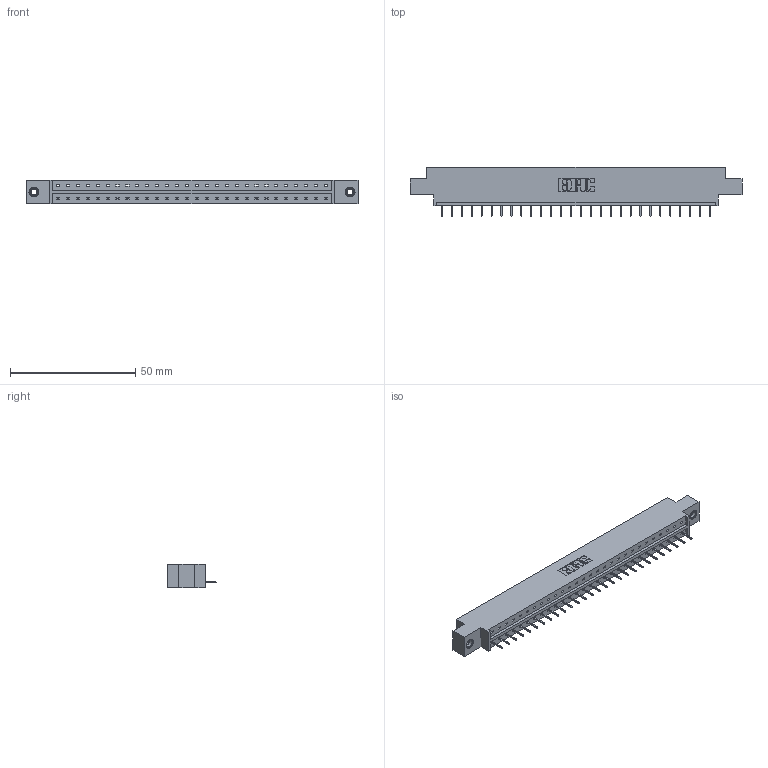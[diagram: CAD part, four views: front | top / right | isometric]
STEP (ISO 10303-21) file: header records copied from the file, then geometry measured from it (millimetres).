
FILE_DESCRIPTION (( 'STEP AP203' ), '1' );
FILE_NAME ('333-028-524-608.STEP', '2018-08-02T14:56:13', ( '' ), ( '' ), 'SwSTEP 2.0', 'SolidWorks 2016', '' );
FILE_SCHEMA (( 'CONFIG_CONTROL_DESIGN' ));
Length unit declared in the file: inch
Products named in the file (4): 333 Part_Offset - .156 Dia - TI; 345-292-001_345-293-124; 345-250-001_345-250-003-102; 333-028-524-608
Assembly tree (31 placements, depth 2):
  333-028-524-608
    333 Part_Offset - .156 Dia - TI
    345-292-001_345-293-124  x28
    345-250-001_345-250-003-102  x2
Bounding box: 132.49 x 19.69 x 9.4 mm (x, y, z)
Volume: 12866.6 mm3; surface area: 13673.5 mm2
Topology: 31 solids, 31 shells, 1914 faces, 5499 edges, 3546 vertices
Faces by surface type: plane 1450, cylinder 448, cone 12, torus 4
Entity records: 20320 total; most frequent: CARTESIAN_POINT 3489, ORIENTED_EDGE 3446, DIRECTION 3005, EDGE_CURVE 1723, VECTOR 1579, LINE 1579, VERTEX_POINT 1140, AXIS2_PLACEMENT_3D 713
